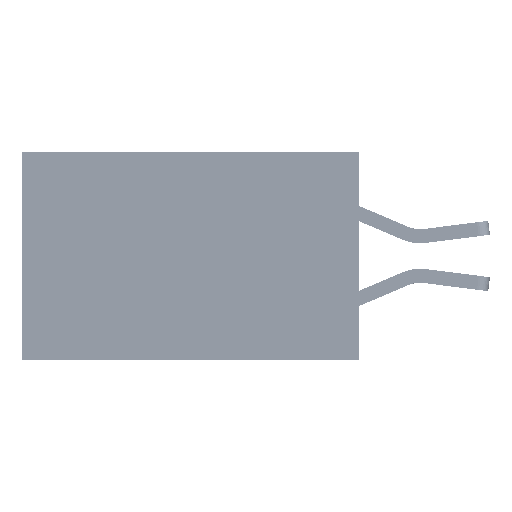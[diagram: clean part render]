
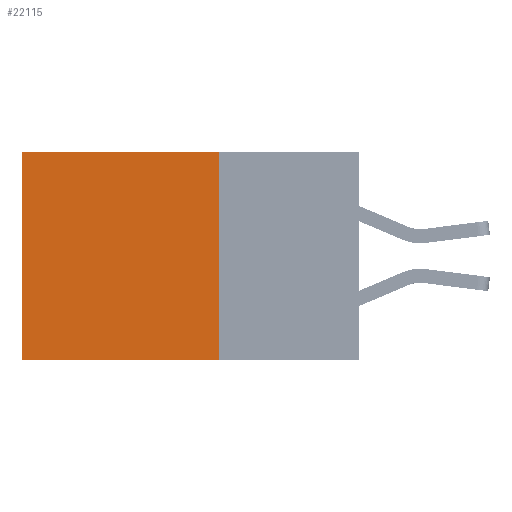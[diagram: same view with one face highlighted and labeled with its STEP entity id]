
A CAD part, left-side view. The second image highlights one B-rep face of the part: STEP entity #22115.
In plain terms, the highlighted planar face has unit normal (-1, 0, 0).
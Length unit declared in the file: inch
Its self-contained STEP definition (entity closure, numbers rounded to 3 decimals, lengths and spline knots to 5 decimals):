
#3499 = VECTOR ( 'NONE', #32502, 39.37008 ) ;
#3725 = CARTESIAN_POINT ( 'NONE',  ( 0.2875, 0.25, -0.37 ) ) ;
#3829 = CARTESIAN_POINT ( 'NONE',  ( 0.2875, 0.25, 0. ) ) ;
#5233 = VECTOR ( 'NONE', #13337, 39.37008 ) ;
#5938 = CARTESIAN_POINT ( 'NONE',  ( 0.2875, 0.6, 0. ) ) ;
#6025 = LINE ( 'NONE', #3725, #3499 ) ;
#8318 = CARTESIAN_POINT ( 'NONE',  ( 0.2875, 0.25, 0. ) ) ;
#11467 = DIRECTION ( 'NONE',  ( 1., 0., 0. ) ) ;
#11602 = DIRECTION ( 'NONE',  ( 0., 0., -1. ) ) ;
#12432 = ORIENTED_EDGE ( 'NONE', *, *, #29911, .F. ) ;
#12468 = AXIS2_PLACEMENT_3D ( 'NONE', #8318, #11467, #11602 ) ;
#13056 = CARTESIAN_POINT ( 'NONE',  ( 0.2875, 0.25, -0.37 ) ) ;
#13337 = DIRECTION ( 'NONE',  ( 0., 0., -1. ) ) ;
#16209 = VERTEX_POINT ( 'NONE', #18630 ) ;
#16481 = LINE ( 'NONE', #26609, #5233 ) ;
#16959 = DIRECTION ( 'NONE',  ( 0., 1., 0. ) ) ;
#17649 = LINE ( 'NONE', #26720, #27395 ) ;
#18245 = EDGE_CURVE ( 'NONE', #16209, #35213, #16481, .T. ) ;
#18630 = CARTESIAN_POINT ( 'NONE',  ( 0.2875, 0.25, 0. ) ) ;
#20223 = CARTESIAN_POINT ( 'NONE',  ( 0.2875, 0.6, -0.37 ) ) ;
#20381 = VECTOR ( 'NONE', #16959, 39.37008 ) ;
#22115 = ADVANCED_FACE ( 'NONE', ( #26842 ), #34086, .F. ) ;
#25577 = VERTEX_POINT ( 'NONE', #5938 ) ;
#26370 = EDGE_CURVE ( 'NONE', #16209, #25577, #29068, .T. ) ;
#26437 = DIRECTION ( 'NONE',  ( 0., 0., -1. ) ) ;
#26609 = CARTESIAN_POINT ( 'NONE',  ( 0.2875, 0.25, 0. ) ) ;
#26720 = CARTESIAN_POINT ( 'NONE',  ( 0.2875, 0.6, 0. ) ) ;
#26842 = FACE_OUTER_BOUND ( 'NONE', #42246, .T. ) ;
#26964 = ORIENTED_EDGE ( 'NONE', *, *, #18245, .F. ) ;
#27395 = VECTOR ( 'NONE', #26437, 39.37008 ) ;
#29023 = ORIENTED_EDGE ( 'NONE', *, *, #38156, .T. ) ;
#29068 = LINE ( 'NONE', #3829, #20381 ) ;
#29911 = EDGE_CURVE ( 'NONE', #35213, #40768, #6025, .T. ) ;
#30596 = ORIENTED_EDGE ( 'NONE', *, *, #26370, .T. ) ;
#32502 = DIRECTION ( 'NONE',  ( 0., 1., 0. ) ) ;
#34086 = PLANE ( 'NONE',  #12468 ) ;
#35213 = VERTEX_POINT ( 'NONE', #13056 ) ;
#38156 = EDGE_CURVE ( 'NONE', #25577, #40768, #17649, .T. ) ;
#40768 = VERTEX_POINT ( 'NONE', #20223 ) ;
#42246 = EDGE_LOOP ( 'NONE', ( #29023, #12432, #26964, #30596 ) ) ;
